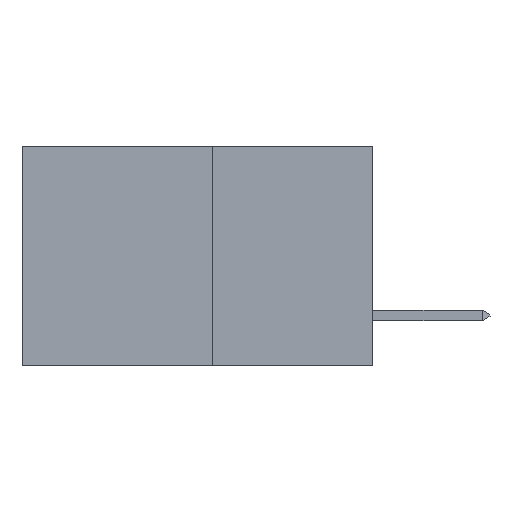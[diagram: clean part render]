
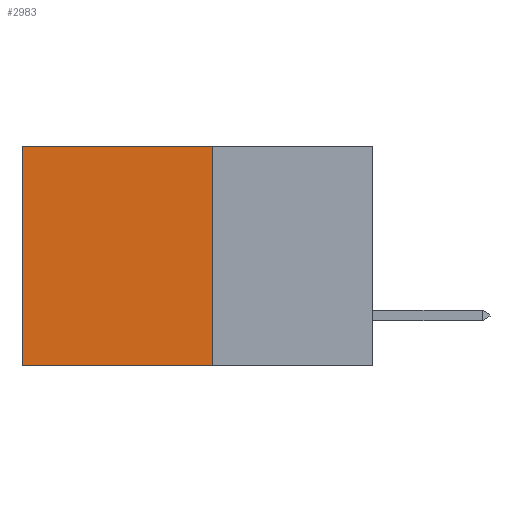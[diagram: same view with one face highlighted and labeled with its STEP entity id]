
A CAD part, left-side view. The second image highlights one B-rep face of the part: STEP entity #2983.
In plain terms, the highlighted planar face has unit normal (-1, 0, 0).
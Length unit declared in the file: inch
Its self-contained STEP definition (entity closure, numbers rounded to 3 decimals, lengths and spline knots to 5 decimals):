
#101 = AXIS2_PLACEMENT_3D ( 'NONE', #9251, #2231, #5487 ) ;
#200 = VERTEX_POINT ( 'NONE', #7111 ) ;
#208 = EDGE_LOOP ( 'NONE', ( #9052, #9504, #9027, #4801 ) ) ;
#527 = DIRECTION ( 'NONE',  ( 0., 0., -1. ) ) ;
#1002 = CARTESIAN_POINT ( 'NONE',  ( 0.277, 0.27, -0.37 ) ) ;
#1102 = LINE ( 'NONE', #1002, #7365 ) ;
#1442 = VERTEX_POINT ( 'NONE', #4889 ) ;
#1625 = CARTESIAN_POINT ( 'NONE',  ( 0.277, 0.27, 0. ) ) ;
#1982 = LINE ( 'NONE', #5214, #6448 ) ;
#1993 = PLANE ( 'NONE',  #101 ) ;
#2040 = FACE_OUTER_BOUND ( 'NONE', #208, .T. ) ;
#2192 = EDGE_CURVE ( 'NONE', #7746, #1442, #3279, .T. ) ;
#2231 = DIRECTION ( 'NONE',  ( 1., 0., 0. ) ) ;
#2983 = ADVANCED_FACE ( 'NONE', ( #2040 ), #1993, .F. ) ;
#3189 = DIRECTION ( 'NONE',  ( 0., 0., -1. ) ) ;
#3279 = LINE ( 'NONE', #5728, #9181 ) ;
#3307 = VECTOR ( 'NONE', #527, 39.37008 ) ;
#3331 = CARTESIAN_POINT ( 'NONE',  ( 0.277, 0.59, 0. ) ) ;
#4356 = DIRECTION ( 'NONE',  ( 0., 1., 0. ) ) ;
#4801 = ORIENTED_EDGE ( 'NONE', *, *, #5758, .T. ) ;
#4889 = CARTESIAN_POINT ( 'NONE',  ( 0.277, 0.27, -0.37 ) ) ;
#5214 = CARTESIAN_POINT ( 'NONE',  ( 0.277, 0.27, 0. ) ) ;
#5487 = DIRECTION ( 'NONE',  ( 0., 0., -1. ) ) ;
#5728 = CARTESIAN_POINT ( 'NONE',  ( 0.277, 0.27, -0.37 ) ) ;
#5758 = EDGE_CURVE ( 'NONE', #7746, #9987, #1982, .T. ) ;
#6448 = VECTOR ( 'NONE', #4356, 39.37008 ) ;
#6534 = DIRECTION ( 'NONE',  ( 0., 1., 0. ) ) ;
#6829 = EDGE_CURVE ( 'NONE', #1442, #200, #1102, .T. ) ;
#7006 = LINE ( 'NONE', #9770, #3307 ) ;
#7111 = CARTESIAN_POINT ( 'NONE',  ( 0.277, 0.59, -0.37 ) ) ;
#7365 = VECTOR ( 'NONE', #6534, 39.37008 ) ;
#7503 = EDGE_CURVE ( 'NONE', #9987, #200, #7006, .T. ) ;
#7746 = VERTEX_POINT ( 'NONE', #1625 ) ;
#9027 = ORIENTED_EDGE ( 'NONE', *, *, #2192, .F. ) ;
#9052 = ORIENTED_EDGE ( 'NONE', *, *, #7503, .T. ) ;
#9181 = VECTOR ( 'NONE', #3189, 39.37008 ) ;
#9251 = CARTESIAN_POINT ( 'NONE',  ( 0.277, 0.27, -0.37 ) ) ;
#9504 = ORIENTED_EDGE ( 'NONE', *, *, #6829, .F. ) ;
#9770 = CARTESIAN_POINT ( 'NONE',  ( 0.277, 0.59, -0.37 ) ) ;
#9987 = VERTEX_POINT ( 'NONE', #3331 ) ;
